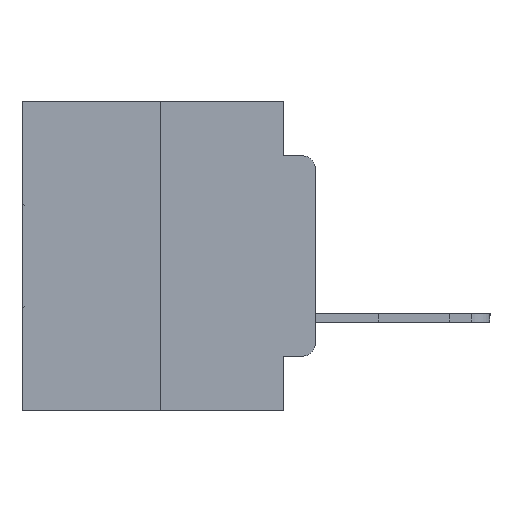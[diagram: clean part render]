
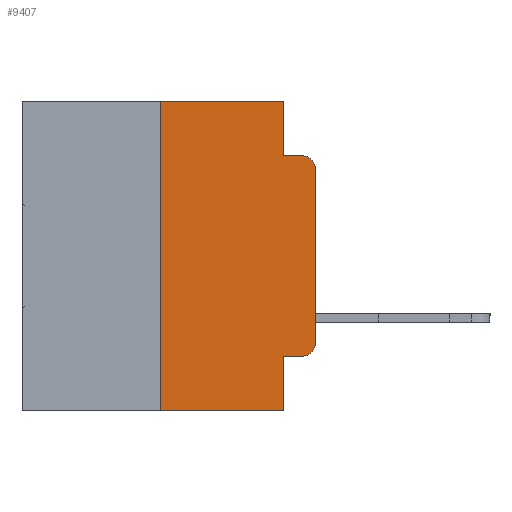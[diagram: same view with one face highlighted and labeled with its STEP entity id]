
A CAD part, left-side view. The second image highlights one B-rep face of the part: STEP entity #9407.
In plain terms, the highlighted planar face has unit normal (-1, 0, 0).
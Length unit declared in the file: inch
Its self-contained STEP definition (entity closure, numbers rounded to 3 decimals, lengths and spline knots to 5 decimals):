
#84 = CARTESIAN_POINT ( 'NONE',  ( 0., 0.473, 0. ) ) ;
#859 = VECTOR ( 'NONE', #26824, 39.37008 ) ;
#1563 = VERTEX_POINT ( 'NONE', #23019 ) ;
#1576 = LINE ( 'NONE', #20144, #859 ) ;
#1750 = EDGE_LOOP ( 'NONE', ( #27979, #11255, #18594, #24210, #14429, #12687, #14788, #11680, #1762, #15137 ) ) ;
#1762 = ORIENTED_EDGE ( 'NONE', *, *, #19949, .T. ) ;
#2403 = DIRECTION ( 'NONE',  ( 0., 0., -1. ) ) ;
#2547 = LINE ( 'NONE', #5531, #13833 ) ;
#2656 = EDGE_CURVE ( 'NONE', #15860, #3787, #11016, .T. ) ;
#2722 = CARTESIAN_POINT ( 'NONE',  ( 0., 0.25, 0. ) ) ;
#3143 = DIRECTION ( 'NONE',  ( 0., 0., 1. ) ) ;
#3343 = EDGE_CURVE ( 'NONE', #7158, #11771, #20419, .T. ) ;
#3507 = CARTESIAN_POINT ( 'NONE',  ( 0., 0., -0.3915 ) ) ;
#3666 = AXIS2_PLACEMENT_3D ( 'NONE', #8519, #24207, #10805 ) ;
#3742 = EDGE_CURVE ( 'NONE', #4979, #22529, #3880, .T. ) ;
#3787 = VERTEX_POINT ( 'NONE', #24568 ) ;
#3877 = LINE ( 'NONE', #13449, #26978 ) ;
#3880 = LINE ( 'NONE', #5645, #26980 ) ;
#4486 = DIRECTION ( 'NONE',  ( 0., -1., 0. ) ) ;
#4741 = EDGE_CURVE ( 'NONE', #8125, #7158, #18918, .T. ) ;
#4948 = CARTESIAN_POINT ( 'NONE',  ( 0., 0.051, 0. ) ) ;
#4979 = VERTEX_POINT ( 'NONE', #15212 ) ;
#5531 = CARTESIAN_POINT ( 'NONE',  ( 0., 0.473, 0. ) ) ;
#5645 = CARTESIAN_POINT ( 'NONE',  ( 0., 0.051, 0. ) ) ;
#5834 = VECTOR ( 'NONE', #26817, 39.37008 ) ;
#5898 = VECTOR ( 'NONE', #17354, 39.37008 ) ;
#7158 = VERTEX_POINT ( 'NONE', #3507 ) ;
#7260 = EDGE_CURVE ( 'NONE', #1563, #22529, #28271, .T. ) ;
#7666 = CARTESIAN_POINT ( 'NONE',  ( 0., 0.02, -0.3915 ) ) ;
#8125 = VERTEX_POINT ( 'NONE', #9284 ) ;
#8404 = CIRCLE ( 'NONE', #3666, 0.02 ) ;
#8418 = CARTESIAN_POINT ( 'NONE',  ( 0., 0.473, -0.5 ) ) ;
#8473 = VECTOR ( 'NONE', #3143, 39.37008 ) ;
#8519 = CARTESIAN_POINT ( 'NONE',  ( 0., 0.02, -0.1085 ) ) ;
#8839 = VERTEX_POINT ( 'NONE', #2722 ) ;
#9284 = CARTESIAN_POINT ( 'NONE',  ( 0., 0.02, -0.4115 ) ) ;
#9407 = ADVANCED_FACE ( 'NONE', ( #12478 ), #13635, .F. ) ;
#9633 = VERTEX_POINT ( 'NONE', #17180 ) ;
#9943 = DIRECTION ( 'NONE',  ( 0., 0., -1. ) ) ;
#10805 = DIRECTION ( 'NONE',  ( 0., 0., -1. ) ) ;
#10894 = EDGE_CURVE ( 'NONE', #8839, #15860, #2547, .T. ) ;
#11016 = LINE ( 'NONE', #4948, #12424 ) ;
#11255 = ORIENTED_EDGE ( 'NONE', *, *, #16538, .T. ) ;
#11680 = ORIENTED_EDGE ( 'NONE', *, *, #3742, .F. ) ;
#11771 = VERTEX_POINT ( 'NONE', #13658 ) ;
#12424 = VECTOR ( 'NONE', #19283, 39.37008 ) ;
#12478 = FACE_OUTER_BOUND ( 'NONE', #1750, .T. ) ;
#12687 = ORIENTED_EDGE ( 'NONE', *, *, #18192, .F. ) ;
#13449 = CARTESIAN_POINT ( 'NONE',  ( 0., 0.051, -0.0885 ) ) ;
#13635 = PLANE ( 'NONE',  #26610 ) ;
#13658 = CARTESIAN_POINT ( 'NONE',  ( 0., 0., -0.1085 ) ) ;
#13833 = VECTOR ( 'NONE', #25715, 39.37008 ) ;
#14429 = ORIENTED_EDGE ( 'NONE', *, *, #10894, .F. ) ;
#14788 = ORIENTED_EDGE ( 'NONE', *, *, #7260, .T. ) ;
#15137 = ORIENTED_EDGE ( 'NONE', *, *, #4741, .T. ) ;
#15212 = CARTESIAN_POINT ( 'NONE',  ( 0., 0.051, -0.4115 ) ) ;
#15860 = VERTEX_POINT ( 'NONE', #25700 ) ;
#15876 = DIRECTION ( 'NONE',  ( 1., 0., 0. ) ) ;
#16538 = EDGE_CURVE ( 'NONE', #11771, #9633, #8404, .T. ) ;
#16634 = AXIS2_PLACEMENT_3D ( 'NONE', #7666, #23354, #9943 ) ;
#17180 = CARTESIAN_POINT ( 'NONE',  ( 0., 0.02, -0.0885 ) ) ;
#17354 = DIRECTION ( 'NONE',  ( 0., -1., 0. ) ) ;
#18192 = EDGE_CURVE ( 'NONE', #1563, #8839, #28214, .T. ) ;
#18594 = ORIENTED_EDGE ( 'NONE', *, *, #26750, .F. ) ;
#18701 = DIRECTION ( 'NONE',  ( 0., 0., -1. ) ) ;
#18918 = CIRCLE ( 'NONE', #16634, 0.02 ) ;
#19283 = DIRECTION ( 'NONE',  ( 0., 0., -1. ) ) ;
#19949 = EDGE_CURVE ( 'NONE', #4979, #8125, #1576, .T. ) ;
#20144 = CARTESIAN_POINT ( 'NONE',  ( 0., 0.051, -0.4115 ) ) ;
#20419 = LINE ( 'NONE', #27311, #8473 ) ;
#22389 = CARTESIAN_POINT ( 'NONE',  ( 0., 0.25, 0. ) ) ;
#22529 = VERTEX_POINT ( 'NONE', #25088 ) ;
#23019 = CARTESIAN_POINT ( 'NONE',  ( 0., 0.25, -0.5 ) ) ;
#23354 = DIRECTION ( 'NONE',  ( -1., 0., 0. ) ) ;
#24207 = DIRECTION ( 'NONE',  ( -1., 0., 0. ) ) ;
#24210 = ORIENTED_EDGE ( 'NONE', *, *, #2656, .F. ) ;
#24568 = CARTESIAN_POINT ( 'NONE',  ( 0., 0.051, -0.0885 ) ) ;
#25088 = CARTESIAN_POINT ( 'NONE',  ( 0., 0.051, -0.5 ) ) ;
#25700 = CARTESIAN_POINT ( 'NONE',  ( 0., 0.051, 0. ) ) ;
#25715 = DIRECTION ( 'NONE',  ( 0., -1., 0. ) ) ;
#26610 = AXIS2_PLACEMENT_3D ( 'NONE', #84, #15876, #2403 ) ;
#26750 = EDGE_CURVE ( 'NONE', #3787, #9633, #3877, .T. ) ;
#26817 = DIRECTION ( 'NONE',  ( 0., 0., 1. ) ) ;
#26824 = DIRECTION ( 'NONE',  ( 0., -1., 0. ) ) ;
#26978 = VECTOR ( 'NONE', #4486, 39.37008 ) ;
#26980 = VECTOR ( 'NONE', #18701, 39.37008 ) ;
#27311 = CARTESIAN_POINT ( 'NONE',  ( 0., 0., 0. ) ) ;
#27979 = ORIENTED_EDGE ( 'NONE', *, *, #3343, .T. ) ;
#28214 = LINE ( 'NONE', #22389, #5834 ) ;
#28271 = LINE ( 'NONE', #8418, #5898 ) ;
